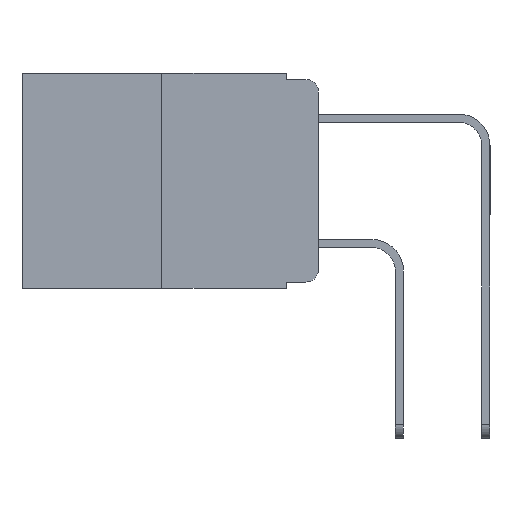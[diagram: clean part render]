
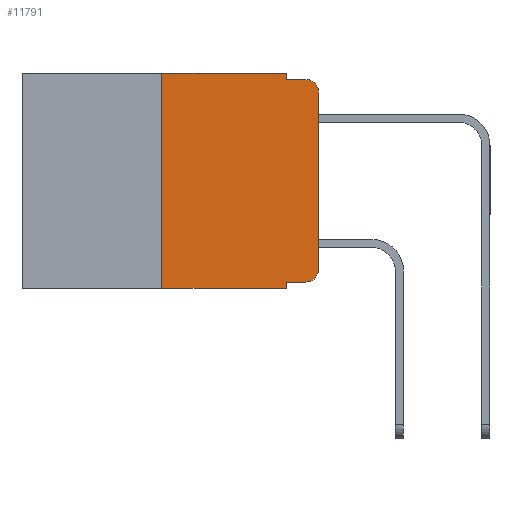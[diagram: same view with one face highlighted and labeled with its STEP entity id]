
A CAD part, left-side view. The second image highlights one B-rep face of the part: STEP entity #11791.
In plain terms, the highlighted planar face has unit normal (-1, 0, 0).
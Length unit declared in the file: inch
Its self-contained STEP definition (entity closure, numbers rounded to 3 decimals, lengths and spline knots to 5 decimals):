
#90 = ORIENTED_EDGE ( 'NONE', *, *, #6089, .F. ) ;
#204 = ORIENTED_EDGE ( 'NONE', *, *, #16262, .T. ) ;
#515 = CARTESIAN_POINT ( 'NONE',  ( 0., 0.25, 0. ) ) ;
#593 = CIRCLE ( 'NONE', #18264, 0.02 ) ;
#1004 = DIRECTION ( 'NONE',  ( 0., -1., 0. ) ) ;
#1914 = EDGE_CURVE ( 'NONE', #11476, #4180, #15143, .T. ) ;
#1993 = DIRECTION ( 'NONE',  ( 0., 0., -1. ) ) ;
#2031 = CARTESIAN_POINT ( 'NONE',  ( 0., 0., -0.03 ) ) ;
#2572 = ORIENTED_EDGE ( 'NONE', *, *, #16912, .T. ) ;
#2623 = LINE ( 'NONE', #19750, #6720 ) ;
#2634 = VERTEX_POINT ( 'NONE', #9441 ) ;
#2658 = EDGE_LOOP ( 'NONE', ( #12665, #12874, #90, #16539, #18064, #3672, #204, #5262, #3169, #2572 ) ) ;
#3169 = ORIENTED_EDGE ( 'NONE', *, *, #16500, .T. ) ;
#3354 = EDGE_CURVE ( 'NONE', #14249, #4637, #19627, .T. ) ;
#3517 = VERTEX_POINT ( 'NONE', #515 ) ;
#3672 = ORIENTED_EDGE ( 'NONE', *, *, #18422, .F. ) ;
#4166 = VERTEX_POINT ( 'NONE', #18321 ) ;
#4180 = VERTEX_POINT ( 'NONE', #2031 ) ;
#4502 = VECTOR ( 'NONE', #6185, 39.37008 ) ;
#4637 = VERTEX_POINT ( 'NONE', #19122 ) ;
#5262 = ORIENTED_EDGE ( 'NONE', *, *, #19848, .F. ) ;
#5632 = CARTESIAN_POINT ( 'NONE',  ( 0., 0.02, -0.313 ) ) ;
#5667 = FACE_OUTER_BOUND ( 'NONE', #2658, .T. ) ;
#5882 = AXIS2_PLACEMENT_3D ( 'NONE', #8748, #12068, #1993 ) ;
#6089 = EDGE_CURVE ( 'NONE', #4637, #4166, #9466, .T. ) ;
#6185 = DIRECTION ( 'NONE',  ( 0., 0., -1. ) ) ;
#6632 = CARTESIAN_POINT ( 'NONE',  ( 0., 0.02, -0.333 ) ) ;
#6720 = VECTOR ( 'NONE', #12032, 39.37008 ) ;
#7078 = VECTOR ( 'NONE', #18335, 39.37008 ) ;
#7190 = EDGE_CURVE ( 'NONE', #4180, #4166, #7823, .T. ) ;
#7348 = DIRECTION ( 'NONE',  ( 0., 0., -1. ) ) ;
#7584 = LINE ( 'NONE', #18457, #15556 ) ;
#7823 = CIRCLE ( 'NONE', #8449, 0.02 ) ;
#8008 = LINE ( 'NONE', #10054, #14986 ) ;
#8449 = AXIS2_PLACEMENT_3D ( 'NONE', #10009, #20964, #11671 ) ;
#8748 = CARTESIAN_POINT ( 'NONE',  ( 0., 0.473, 0. ) ) ;
#9441 = CARTESIAN_POINT ( 'NONE',  ( 0., 0.051, -0.333 ) ) ;
#9466 = LINE ( 'NONE', #17175, #17358 ) ;
#9595 = CARTESIAN_POINT ( 'NONE',  ( 0., 0.051, -0.333 ) ) ;
#10009 = CARTESIAN_POINT ( 'NONE',  ( 0., 0.02, -0.03 ) ) ;
#10054 = CARTESIAN_POINT ( 'NONE',  ( 0., 0.25, 0. ) ) ;
#10413 = VECTOR ( 'NONE', #11901, 39.37008 ) ;
#10679 = DIRECTION ( 'NONE',  ( 0., -1., 0. ) ) ;
#10969 = CARTESIAN_POINT ( 'NONE',  ( 0., 0.25, -0.343 ) ) ;
#11383 = CARTESIAN_POINT ( 'NONE',  ( 0., 0.051, -0.343 ) ) ;
#11476 = VERTEX_POINT ( 'NONE', #19042 ) ;
#11671 = DIRECTION ( 'NONE',  ( 0., 0., -1. ) ) ;
#11708 = DIRECTION ( 'NONE',  ( 0., 0., 1. ) ) ;
#11791 = ADVANCED_FACE ( 'NONE', ( #5667 ), #19793, .F. ) ;
#11901 = DIRECTION ( 'NONE',  ( 0., 0., 1. ) ) ;
#12032 = DIRECTION ( 'NONE',  ( 0., -1., 0. ) ) ;
#12068 = DIRECTION ( 'NONE',  ( 1., 0., 0. ) ) ;
#12620 = EDGE_CURVE ( 'NONE', #3517, #14249, #2623, .T. ) ;
#12665 = ORIENTED_EDGE ( 'NONE', *, *, #1914, .T. ) ;
#12874 = ORIENTED_EDGE ( 'NONE', *, *, #7190, .T. ) ;
#12909 = CARTESIAN_POINT ( 'NONE',  ( 0., 0.051, 0. ) ) ;
#13217 = LINE ( 'NONE', #20419, #4502 ) ;
#14249 = VERTEX_POINT ( 'NONE', #12909 ) ;
#14986 = VECTOR ( 'NONE', #11708, 39.37008 ) ;
#15143 = LINE ( 'NONE', #19624, #10413 ) ;
#15274 = CARTESIAN_POINT ( 'NONE',  ( 0., 0.051, 0. ) ) ;
#15556 = VECTOR ( 'NONE', #10679, 39.37008 ) ;
#15793 = VECTOR ( 'NONE', #1004, 39.37008 ) ;
#16262 = EDGE_CURVE ( 'NONE', #16336, #19983, #7584, .T. ) ;
#16270 = LINE ( 'NONE', #9595, #15793 ) ;
#16336 = VERTEX_POINT ( 'NONE', #10969 ) ;
#16500 = EDGE_CURVE ( 'NONE', #2634, #16592, #16270, .T. ) ;
#16539 = ORIENTED_EDGE ( 'NONE', *, *, #3354, .F. ) ;
#16592 = VERTEX_POINT ( 'NONE', #6632 ) ;
#16835 = DIRECTION ( 'NONE',  ( -1., 0., 0. ) ) ;
#16912 = EDGE_CURVE ( 'NONE', #16592, #11476, #593, .T. ) ;
#17175 = CARTESIAN_POINT ( 'NONE',  ( 0., 0.051, -0.01 ) ) ;
#17358 = VECTOR ( 'NONE', #18701, 39.37008 ) ;
#18064 = ORIENTED_EDGE ( 'NONE', *, *, #12620, .F. ) ;
#18264 = AXIS2_PLACEMENT_3D ( 'NONE', #5632, #16835, #7348 ) ;
#18321 = CARTESIAN_POINT ( 'NONE',  ( 0., 0.02, -0.01 ) ) ;
#18335 = DIRECTION ( 'NONE',  ( 0., 0., -1. ) ) ;
#18422 = EDGE_CURVE ( 'NONE', #16336, #3517, #8008, .T. ) ;
#18457 = CARTESIAN_POINT ( 'NONE',  ( 0., 0.473, -0.343 ) ) ;
#18701 = DIRECTION ( 'NONE',  ( 0., -1., 0. ) ) ;
#19042 = CARTESIAN_POINT ( 'NONE',  ( 0., 0., -0.313 ) ) ;
#19122 = CARTESIAN_POINT ( 'NONE',  ( 0., 0.051, -0.01 ) ) ;
#19624 = CARTESIAN_POINT ( 'NONE',  ( 0., 0., 0. ) ) ;
#19627 = LINE ( 'NONE', #15274, #7078 ) ;
#19750 = CARTESIAN_POINT ( 'NONE',  ( 0., 0.473, 0. ) ) ;
#19793 = PLANE ( 'NONE',  #5882 ) ;
#19848 = EDGE_CURVE ( 'NONE', #2634, #19983, #13217, .T. ) ;
#19983 = VERTEX_POINT ( 'NONE', #11383 ) ;
#20419 = CARTESIAN_POINT ( 'NONE',  ( 0., 0.051, 0. ) ) ;
#20964 = DIRECTION ( 'NONE',  ( -1., 0., 0. ) ) ;
